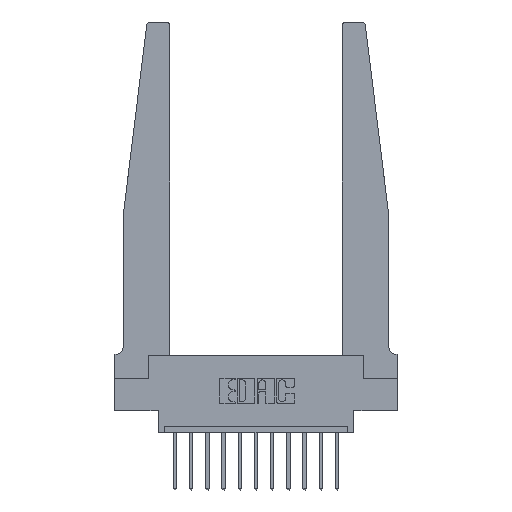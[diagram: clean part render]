
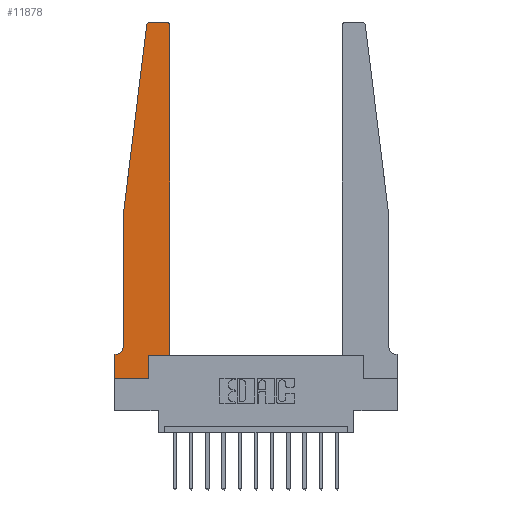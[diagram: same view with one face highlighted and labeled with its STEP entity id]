
A CAD part, top view. The second image highlights one B-rep face of the part: STEP entity #11878.
In plain terms, the highlighted planar face has unit normal (0, 0, 1).
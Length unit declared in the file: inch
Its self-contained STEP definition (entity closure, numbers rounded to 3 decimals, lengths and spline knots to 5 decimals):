
#119 = VERTEX_POINT ( 'NONE', #15010 ) ;
#126 = VERTEX_POINT ( 'NONE', #3682 ) ;
#194 = CARTESIAN_POINT ( 'NONE',  ( 0.2605, 0.18, 0.37 ) ) ;
#699 = CIRCLE ( 'NONE', #958, 0.03 ) ;
#733 = CARTESIAN_POINT ( 'NONE',  ( 0.27653, 2.75, 0.37 ) ) ;
#904 = DIRECTION ( 'NONE',  ( 0., -1., 0. ) ) ;
#958 = AXIS2_PLACEMENT_3D ( 'NONE', #3411, #12344, #8456 ) ;
#1009 = CARTESIAN_POINT ( 'NONE',  ( 0.425, 0.18, 0.37 ) ) ;
#1435 = CARTESIAN_POINT ( 'NONE',  ( 0.015, 0.2375, 0.37 ) ) ;
#1556 = VECTOR ( 'NONE', #904, 39.37008 ) ;
#1594 = DIRECTION ( 'NONE',  ( -1., 0., 0. ) ) ;
#1695 = ORIENTED_EDGE ( 'NONE', *, *, #10843, .T. ) ;
#1813 = AXIS2_PLACEMENT_3D ( 'NONE', #1435, #2661, #1594 ) ;
#1830 = ORIENTED_EDGE ( 'NONE', *, *, #7477, .T. ) ;
#2073 = EDGE_CURVE ( 'NONE', #3723, #9957, #6639, .T. ) ;
#2224 = VECTOR ( 'NONE', #5247, 39.37008 ) ;
#2595 = CARTESIAN_POINT ( 'NONE',  ( 0., 0., 0.37 ) ) ;
#2661 = DIRECTION ( 'NONE',  ( 0., 0., -1. ) ) ;
#2681 = LINE ( 'NONE', #9306, #4962 ) ;
#2985 = ORIENTED_EDGE ( 'NONE', *, *, #2073, .T. ) ;
#3017 = DIRECTION ( 'NONE',  ( 1., 0., 0. ) ) ;
#3411 = CARTESIAN_POINT ( 'NONE',  ( 0.27653, 2.72, 0.37 ) ) ;
#3418 = ORIENTED_EDGE ( 'NONE', *, *, #8215, .T. ) ;
#3483 = CARTESIAN_POINT ( 'NONE',  ( 0.425, 2.72, 0.37 ) ) ;
#3682 = CARTESIAN_POINT ( 'NONE',  ( 0.065, 0.2375, 0.37 ) ) ;
#3723 = VERTEX_POINT ( 'NONE', #10293 ) ;
#3826 = EDGE_CURVE ( 'NONE', #9957, #6632, #14489, .T. ) ;
#3907 = CARTESIAN_POINT ( 'NONE',  ( 0.395, 2.75, 0.37 ) ) ;
#4206 = VERTEX_POINT ( 'NONE', #5213 ) ;
#4317 = DIRECTION ( 'NONE',  ( -1., 0., 0. ) ) ;
#4495 = DIRECTION ( 'NONE',  ( 1., 0., 0. ) ) ;
#4962 = VECTOR ( 'NONE', #9059, 39.37008 ) ;
#5025 = VERTEX_POINT ( 'NONE', #7730 ) ;
#5044 = EDGE_CURVE ( 'NONE', #15846, #5323, #11175, .T. ) ;
#5213 = CARTESIAN_POINT ( 'NONE',  ( 0.065, 1.25, 0.37 ) ) ;
#5247 = DIRECTION ( 'NONE',  ( 1., 0., 0. ) ) ;
#5323 = VERTEX_POINT ( 'NONE', #3907 ) ;
#5569 = CARTESIAN_POINT ( 'NONE',  ( 0., 0.1875, 0.37 ) ) ;
#5595 = VERTEX_POINT ( 'NONE', #14784 ) ;
#5670 = CARTESIAN_POINT ( 'NONE',  ( 0.395, 2.72, 0.37 ) ) ;
#5730 = LINE ( 'NONE', #1009, #7298 ) ;
#5979 = CARTESIAN_POINT ( 'NONE',  ( 0.425, 0.18, 0.37 ) ) ;
#6632 = VERTEX_POINT ( 'NONE', #8983 ) ;
#6639 = LINE ( 'NONE', #13073, #7112 ) ;
#6864 = CARTESIAN_POINT ( 'NONE',  ( 0.065, 1.25, 0.37 ) ) ;
#7112 = VECTOR ( 'NONE', #4317, 39.37008 ) ;
#7298 = VECTOR ( 'NONE', #10781, 39.37008 ) ;
#7477 = EDGE_CURVE ( 'NONE', #5323, #12904, #13732, .T. ) ;
#7484 = ORIENTED_EDGE ( 'NONE', *, *, #15242, .T. ) ;
#7730 = CARTESIAN_POINT ( 'NONE',  ( 0.2605, 0.18, 0.37 ) ) ;
#7781 = EDGE_LOOP ( 'NONE', ( #1830, #10553, #12009, #7484, #11233, #2985, #11993, #3418, #14787, #16093, #1695, #11411 ) ) ;
#8052 = VECTOR ( 'NONE', #11431, 39.37008 ) ;
#8215 = EDGE_CURVE ( 'NONE', #6632, #119, #13922, .T. ) ;
#8431 = CARTESIAN_POINT ( 'NONE',  ( 0.065, 1.25, 0.37 ) ) ;
#8456 = DIRECTION ( 'NONE',  ( 1., 0., 0. ) ) ;
#8957 = DIRECTION ( 'NONE',  ( 0., 1., 0. ) ) ;
#8983 = CARTESIAN_POINT ( 'NONE',  ( 0., 0., 0.37 ) ) ;
#9059 = DIRECTION ( 'NONE',  ( 1., 0., 0. ) ) ;
#9186 = EDGE_CURVE ( 'NONE', #5595, #4206, #9427, .T. ) ;
#9290 = DIRECTION ( 'NONE',  ( 0., 0., 1. ) ) ;
#9306 = CARTESIAN_POINT ( 'NONE',  ( 0.425, 0.18, 0.37 ) ) ;
#9427 = LINE ( 'NONE', #6864, #16237 ) ;
#9476 = DIRECTION ( 'NONE',  ( 0., 0., 1. ) ) ;
#9672 = LINE ( 'NONE', #8431, #1556 ) ;
#9733 = VECTOR ( 'NONE', #8957, 39.37008 ) ;
#9804 = EDGE_CURVE ( 'NONE', #12904, #5595, #699, .T. ) ;
#9957 = VERTEX_POINT ( 'NONE', #12315 ) ;
#10135 = AXIS2_PLACEMENT_3D ( 'NONE', #5670, #9476, #3017 ) ;
#10293 = CARTESIAN_POINT ( 'NONE',  ( 0.015, 0.1875, 0.37 ) ) ;
#10375 = LINE ( 'NONE', #194, #9733 ) ;
#10553 = ORIENTED_EDGE ( 'NONE', *, *, #9804, .T. ) ;
#10781 = DIRECTION ( 'NONE',  ( 0., 1., 0. ) ) ;
#10843 = EDGE_CURVE ( 'NONE', #11976, #15846, #5730, .T. ) ;
#11175 = CIRCLE ( 'NONE', #10135, 0.03 ) ;
#11233 = ORIENTED_EDGE ( 'NONE', *, *, #14474, .T. ) ;
#11264 = CARTESIAN_POINT ( 'NONE',  ( 0.25, 2.75, 0.37 ) ) ;
#11411 = ORIENTED_EDGE ( 'NONE', *, *, #5044, .T. ) ;
#11431 = DIRECTION ( 'NONE',  ( -1., 0., 0. ) ) ;
#11770 = FACE_OUTER_BOUND ( 'NONE', #7781, .T. ) ;
#11878 = ADVANCED_FACE ( 'NONE', ( #11770 ), #15807, .T. ) ;
#11976 = VERTEX_POINT ( 'NONE', #5979 ) ;
#11993 = ORIENTED_EDGE ( 'NONE', *, *, #3826, .T. ) ;
#12009 = ORIENTED_EDGE ( 'NONE', *, *, #9186, .T. ) ;
#12167 = DIRECTION ( 'NONE',  ( 0., -1., 0. ) ) ;
#12315 = CARTESIAN_POINT ( 'NONE',  ( 0., 0.1875, 0.37 ) ) ;
#12344 = DIRECTION ( 'NONE',  ( 0., 0., 1. ) ) ;
#12633 = CIRCLE ( 'NONE', #1813, 0.05 ) ;
#12904 = VERTEX_POINT ( 'NONE', #733 ) ;
#13073 = CARTESIAN_POINT ( 'NONE',  ( 0.065, 0.1875, 0.37 ) ) ;
#13141 = AXIS2_PLACEMENT_3D ( 'NONE', #5569, #9290, #4495 ) ;
#13161 = CARTESIAN_POINT ( 'NONE',  ( 0., 0., 0.37 ) ) ;
#13732 = LINE ( 'NONE', #11264, #8052 ) ;
#13922 = LINE ( 'NONE', #2595, #2224 ) ;
#14057 = EDGE_CURVE ( 'NONE', #5025, #11976, #2681, .T. ) ;
#14466 = DIRECTION ( 'NONE',  ( -0.122, -0.992, 0. ) ) ;
#14474 = EDGE_CURVE ( 'NONE', #126, #3723, #12633, .T. ) ;
#14489 = LINE ( 'NONE', #13161, #15103 ) ;
#14510 = EDGE_CURVE ( 'NONE', #119, #5025, #10375, .T. ) ;
#14784 = CARTESIAN_POINT ( 'NONE',  ( 0.24675, 2.72367, 0.37 ) ) ;
#14787 = ORIENTED_EDGE ( 'NONE', *, *, #14510, .T. ) ;
#15010 = CARTESIAN_POINT ( 'NONE',  ( 0.2605, 0., 0.37 ) ) ;
#15103 = VECTOR ( 'NONE', #12167, 39.37008 ) ;
#15242 = EDGE_CURVE ( 'NONE', #4206, #126, #9672, .T. ) ;
#15807 = PLANE ( 'NONE',  #13141 ) ;
#15846 = VERTEX_POINT ( 'NONE', #3483 ) ;
#16093 = ORIENTED_EDGE ( 'NONE', *, *, #14057, .T. ) ;
#16237 = VECTOR ( 'NONE', #14466, 39.37008 ) ;
